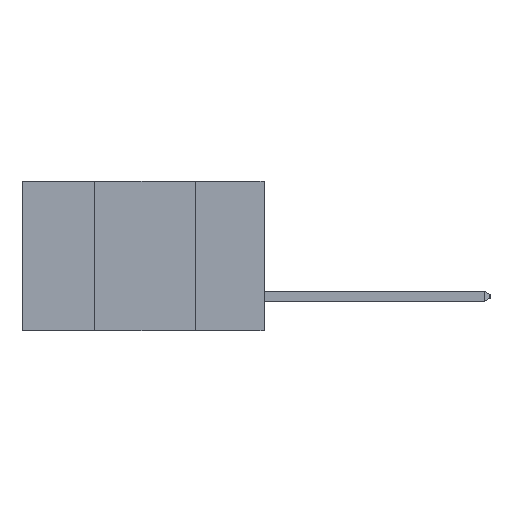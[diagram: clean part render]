
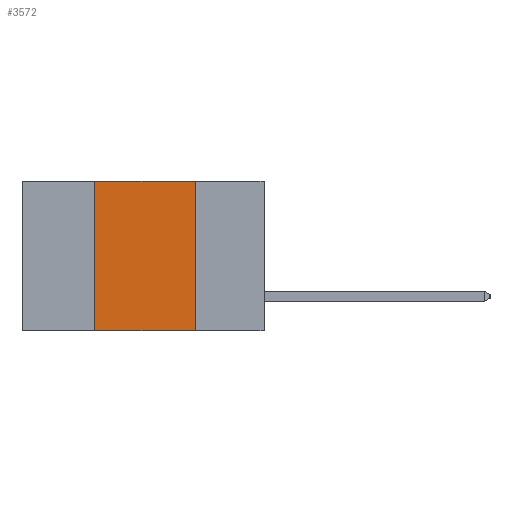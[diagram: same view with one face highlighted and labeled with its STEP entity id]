
A CAD part, left-side view. The second image highlights one B-rep face of the part: STEP entity #3572.
In plain terms, the highlighted planar face has unit normal (-1, 0, 0).
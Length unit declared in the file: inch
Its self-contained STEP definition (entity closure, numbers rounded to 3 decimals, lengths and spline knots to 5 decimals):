
#22 = CARTESIAN_POINT ( 'NONE',  ( 0., 0.17, -0.37 ) ) ;
#410 = VERTEX_POINT ( 'NONE', #8195 ) ;
#1261 = LINE ( 'NONE', #4560, #10989 ) ;
#1474 = DIRECTION ( 'NONE',  ( 0., -1., 0. ) ) ;
#2056 = EDGE_CURVE ( 'NONE', #410, #10529, #3276, .T. ) ;
#2087 = AXIS2_PLACEMENT_3D ( 'NONE', #2311, #9256, #6997 ) ;
#2311 = CARTESIAN_POINT ( 'NONE',  ( 0., 0.6, 0. ) ) ;
#3112 = VERTEX_POINT ( 'NONE', #7888 ) ;
#3276 = LINE ( 'NONE', #10580, #7871 ) ;
#3320 = EDGE_LOOP ( 'NONE', ( #5747, #11416, #9437, #5812 ) ) ;
#3439 = EDGE_CURVE ( 'NONE', #410, #3112, #10044, .T. ) ;
#3572 = ADVANCED_FACE ( 'NONE', ( #4141 ), #9269, .F. ) ;
#3842 = VECTOR ( 'NONE', #10295, 39.37008 ) ;
#4141 = FACE_OUTER_BOUND ( 'NONE', #3320, .T. ) ;
#4424 = EDGE_CURVE ( 'NONE', #3112, #5754, #10719, .T. ) ;
#4560 = CARTESIAN_POINT ( 'NONE',  ( 0., 0.17, -0.37 ) ) ;
#5747 = ORIENTED_EDGE ( 'NONE', *, *, #9984, .F. ) ;
#5754 = VERTEX_POINT ( 'NONE', #8813 ) ;
#5812 = ORIENTED_EDGE ( 'NONE', *, *, #2056, .T. ) ;
#6997 = DIRECTION ( 'NONE',  ( 0., 0., -1. ) ) ;
#7871 = VECTOR ( 'NONE', #1474, 39.37008 ) ;
#7888 = CARTESIAN_POINT ( 'NONE',  ( 0., 0.42, 0. ) ) ;
#8155 = DIRECTION ( 'NONE',  ( 0., 0., -1. ) ) ;
#8195 = CARTESIAN_POINT ( 'NONE',  ( 0., 0.42, -0.37 ) ) ;
#8265 = DIRECTION ( 'NONE',  ( 0., 0., 1. ) ) ;
#8438 = CARTESIAN_POINT ( 'NONE',  ( 0., 0.42, -0.37 ) ) ;
#8813 = CARTESIAN_POINT ( 'NONE',  ( 0., 0.17, 0. ) ) ;
#9256 = DIRECTION ( 'NONE',  ( 1., 0., 0. ) ) ;
#9269 = PLANE ( 'NONE',  #2087 ) ;
#9437 = ORIENTED_EDGE ( 'NONE', *, *, #3439, .F. ) ;
#9984 = EDGE_CURVE ( 'NONE', #5754, #10529, #1261, .T. ) ;
#10044 = LINE ( 'NONE', #8438, #10315 ) ;
#10295 = DIRECTION ( 'NONE',  ( 0., -1., 0. ) ) ;
#10315 = VECTOR ( 'NONE', #8265, 39.37008 ) ;
#10529 = VERTEX_POINT ( 'NONE', #22 ) ;
#10580 = CARTESIAN_POINT ( 'NONE',  ( 0., 0.6, -0.37 ) ) ;
#10719 = LINE ( 'NONE', #11464, #3842 ) ;
#10989 = VECTOR ( 'NONE', #8155, 39.37008 ) ;
#11416 = ORIENTED_EDGE ( 'NONE', *, *, #4424, .F. ) ;
#11464 = CARTESIAN_POINT ( 'NONE',  ( 0., 0.6, 0. ) ) ;
